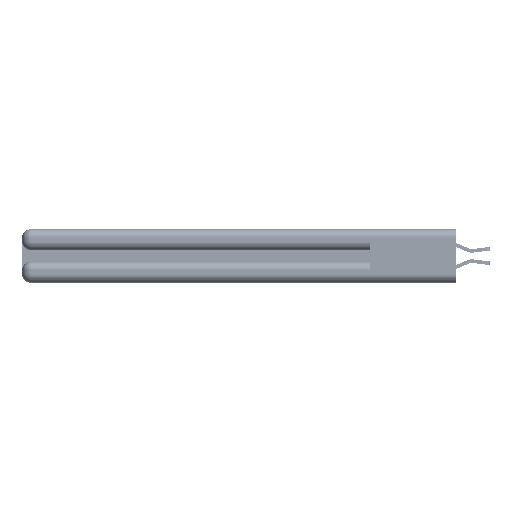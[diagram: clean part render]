
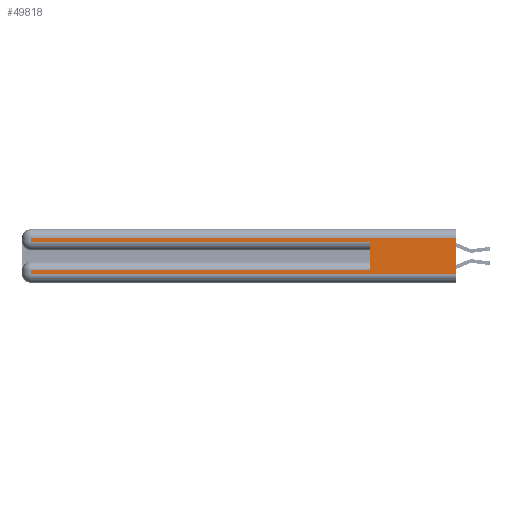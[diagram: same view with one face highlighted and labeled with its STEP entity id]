
A CAD part, left-side view. The second image highlights one B-rep face of the part: STEP entity #49818.
In plain terms, the highlighted planar face has unit normal (-1, 0, 0).
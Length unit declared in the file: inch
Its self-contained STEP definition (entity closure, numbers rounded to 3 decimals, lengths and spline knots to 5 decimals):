
#307 = CARTESIAN_POINT ( 'NONE',  ( 0., 0., 0.31 ) ) ;
#1596 = AXIS2_PLACEMENT_3D ( 'NONE', #37878, #20998, #50493 ) ;
#2184 = EDGE_CURVE ( 'NONE', #21950, #28836, #38041, .T. ) ;
#2354 = CARTESIAN_POINT ( 'NONE',  ( 0., 0., 0.37 ) ) ;
#3340 = DIRECTION ( 'NONE',  ( 0., 0., -1. ) ) ;
#3835 = VECTOR ( 'NONE', #30127, 39.37008 ) ;
#4166 = VECTOR ( 'NONE', #7396, 39.37008 ) ;
#4804 = ORIENTED_EDGE ( 'NONE', *, *, #51385, .T. ) ;
#5465 = VERTEX_POINT ( 'NONE', #19870 ) ;
#5629 = ORIENTED_EDGE ( 'NONE', *, *, #50124, .T. ) ;
#5912 = DIRECTION ( 'NONE',  ( 0., -1., 0. ) ) ;
#6119 = LINE ( 'NONE', #23010, #17388 ) ;
#7396 = DIRECTION ( 'NONE',  ( 0., 1., 0. ) ) ;
#8885 = CARTESIAN_POINT ( 'NONE',  ( 0., 0.6, 0.145 ) ) ;
#9498 = FACE_OUTER_BOUND ( 'NONE', #27443, .T. ) ;
#9991 = LINE ( 'NONE', #37311, #31310 ) ;
#10817 = CARTESIAN_POINT ( 'NONE',  ( 0., 2.94, 0.31 ) ) ;
#10887 = LINE ( 'NONE', #2354, #32193 ) ;
#12482 = VECTOR ( 'NONE', #17361, 39.37008 ) ;
#12531 = VERTEX_POINT ( 'NONE', #34683 ) ;
#13431 = CARTESIAN_POINT ( 'NONE',  ( 0., 2.94, 0.285 ) ) ;
#13804 = LINE ( 'NONE', #307, #3835 ) ;
#14880 = EDGE_CURVE ( 'NONE', #5465, #12531, #51026, .T. ) ;
#16181 = ORIENTED_EDGE ( 'NONE', *, *, #14880, .T. ) ;
#16941 = CARTESIAN_POINT ( 'NONE',  ( 0., 0., 0.06 ) ) ;
#17330 = VECTOR ( 'NONE', #25582, 39.37008 ) ;
#17361 = DIRECTION ( 'NONE',  ( 0., 0., 1. ) ) ;
#17388 = VECTOR ( 'NONE', #5912, 39.37008 ) ;
#17878 = ORIENTED_EDGE ( 'NONE', *, *, #30513, .T. ) ;
#18647 = CARTESIAN_POINT ( 'NONE',  ( 0., 0.6, 0.085 ) ) ;
#19870 = CARTESIAN_POINT ( 'NONE',  ( 0., 2.94, 0.06 ) ) ;
#20511 = CARTESIAN_POINT ( 'NONE',  ( 0., 0., 0.31 ) ) ;
#20998 = DIRECTION ( 'NONE',  ( 1., 0., 0. ) ) ;
#21950 = VERTEX_POINT ( 'NONE', #18647 ) ;
#23010 = CARTESIAN_POINT ( 'NONE',  ( 0., 0., 0.285 ) ) ;
#23221 = CARTESIAN_POINT ( 'NONE',  ( 0., 2.94, 0.37 ) ) ;
#23786 = LINE ( 'NONE', #8885, #12482 ) ;
#25582 = DIRECTION ( 'NONE',  ( 0., -1., 0. ) ) ;
#26585 = EDGE_CURVE ( 'NONE', #42225, #12531, #10887, .T. ) ;
#27412 = VECTOR ( 'NONE', #48645, 39.37008 ) ;
#27443 = EDGE_LOOP ( 'NONE', ( #46541, #45120, #4804, #5629, #53949, #41489, #17878, #16181 ) ) ;
#28836 = VERTEX_POINT ( 'NONE', #45703 ) ;
#30127 = DIRECTION ( 'NONE',  ( 0., 1., 0. ) ) ;
#30513 = EDGE_CURVE ( 'NONE', #28836, #5465, #49730, .T. ) ;
#31310 = VECTOR ( 'NONE', #3340, 39.37008 ) ;
#32193 = VECTOR ( 'NONE', #40421, 39.37008 ) ;
#34683 = CARTESIAN_POINT ( 'NONE',  ( 0., 0., 0.06 ) ) ;
#37086 = CARTESIAN_POINT ( 'NONE',  ( 0., 0., 0.085 ) ) ;
#37311 = CARTESIAN_POINT ( 'NONE',  ( 0., 2.94, 0.37 ) ) ;
#37642 = EDGE_CURVE ( 'NONE', #42225, #53153, #13804, .T. ) ;
#37681 = EDGE_CURVE ( 'NONE', #21950, #48734, #23786, .T. ) ;
#37878 = CARTESIAN_POINT ( 'NONE',  ( 0., 0., 0.37 ) ) ;
#38041 = LINE ( 'NONE', #37086, #4166 ) ;
#40421 = DIRECTION ( 'NONE',  ( 0., 0., -1. ) ) ;
#41489 = ORIENTED_EDGE ( 'NONE', *, *, #2184, .T. ) ;
#42024 = CARTESIAN_POINT ( 'NONE',  ( 0., 0.6, 0.285 ) ) ;
#42225 = VERTEX_POINT ( 'NONE', #20511 ) ;
#45120 = ORIENTED_EDGE ( 'NONE', *, *, #37642, .T. ) ;
#45703 = CARTESIAN_POINT ( 'NONE',  ( 0., 2.94, 0.085 ) ) ;
#46072 = VERTEX_POINT ( 'NONE', #13431 ) ;
#46298 = PLANE ( 'NONE',  #1596 ) ;
#46541 = ORIENTED_EDGE ( 'NONE', *, *, #26585, .F. ) ;
#48645 = DIRECTION ( 'NONE',  ( 0., 0., -1. ) ) ;
#48734 = VERTEX_POINT ( 'NONE', #42024 ) ;
#49730 = LINE ( 'NONE', #23221, #27412 ) ;
#49818 = ADVANCED_FACE ( 'NONE', ( #9498 ), #46298, .F. ) ;
#50124 = EDGE_CURVE ( 'NONE', #46072, #48734, #6119, .T. ) ;
#50493 = DIRECTION ( 'NONE',  ( 0., 0., -1. ) ) ;
#51026 = LINE ( 'NONE', #16941, #17330 ) ;
#51385 = EDGE_CURVE ( 'NONE', #53153, #46072, #9991, .T. ) ;
#53153 = VERTEX_POINT ( 'NONE', #10817 ) ;
#53949 = ORIENTED_EDGE ( 'NONE', *, *, #37681, .F. ) ;
